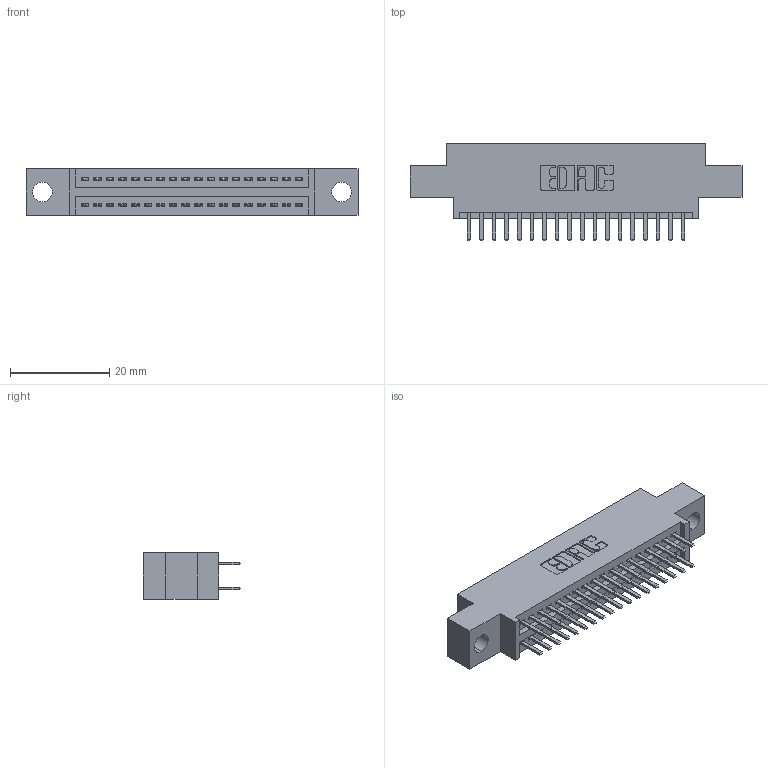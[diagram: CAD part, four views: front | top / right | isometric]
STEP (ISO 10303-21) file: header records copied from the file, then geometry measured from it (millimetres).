
FILE_DESCRIPTION (( 'STEP AP203' ), '1' );
FILE_NAME ('395-036-520-804.STEP', '2021-06-16T21:02:29', ( '' ), ( '' ), 'SwSTEP 2.0', 'SolidWorks 2020', '' );
FILE_SCHEMA (( 'CONFIG_CONTROL_DESIGN' ));
Length unit declared in the file: inch
Products named in the file (3): 345 Part_0.170 Offset - 0.156 Dia-TI; 395-036-520-804; 345-292-001_345-293-120
Assembly tree (37 placements, depth 2):
  395-036-520-804
    345 Part_0.170 Offset - 0.156 Dia-TI
    345-292-001_345-293-120  x36
Bounding box: 66.93 x 19.68 x 9.4 mm (x, y, z)
Volume: 6043.6 mm3; surface area: 8430.1 mm2
Topology: 37 solids, 37 shells, 2088 faces, 6041 edges, 3930 vertices
Faces by surface type: plane 1358, cylinder 730
Entity records: 18019 total; most frequent: CARTESIAN_POINT 3062, ORIENTED_EDGE 2982, DIRECTION 2715, EDGE_CURVE 1491, LINE 1283, VECTOR 1283, VERTEX_POINT 990, AXIS2_PLACEMENT_3D 716
